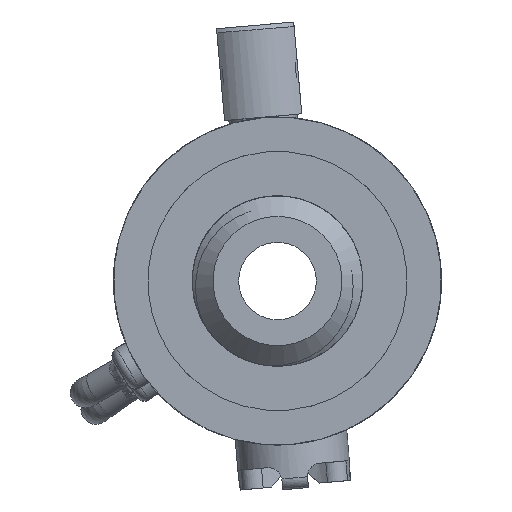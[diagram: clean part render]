
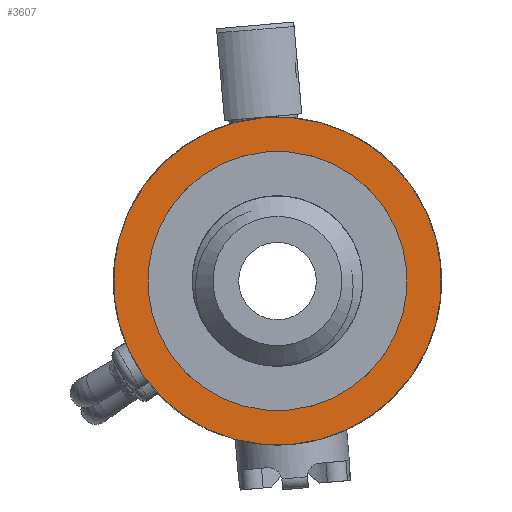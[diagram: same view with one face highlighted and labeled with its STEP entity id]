
A CAD part, left-side view. The second image highlights one B-rep face of the part: STEP entity #3607.
In plain terms, the highlighted planar face has unit normal (-1, 0, 0).
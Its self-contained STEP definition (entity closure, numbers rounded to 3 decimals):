
#204=FACE_BOUND('',#1165,.T.);
#894=FACE_OUTER_BOUND('',#1164,.T.);
#1164=EDGE_LOOP('',(#2832));
#1165=EDGE_LOOP('',(#2833));
#1320=CIRCLE('',#3817,15.05);
#1323=CIRCLE('',#3833,19.05);
#1523=VERTEX_POINT('',#6397);
#1571=VERTEX_POINT('',#7305);
#1927=EDGE_CURVE('',#1523,#1523,#1320,.T.);
#1991=EDGE_CURVE('',#1571,#1571,#1323,.T.);
#2832=ORIENTED_EDGE('',*,*,#1991,.T.);
#2833=ORIENTED_EDGE('',*,*,#1927,.T.);
#3510=PLANE('',#3857);
#3607=ADVANCED_FACE('',(#894,#204),#3510,.T.);
#3817=AXIS2_PLACEMENT_3D('',#6398,#4250,#4251);
#3833=AXIS2_PLACEMENT_3D('',#7306,#4302,#4303);
#3857=AXIS2_PLACEMENT_3D('',#7939,#4367,#4368);
#4250=DIRECTION('center_axis',(1.,0.,0.));
#4251=DIRECTION('ref_axis',(0.,0.996,-0.087));
#4302=DIRECTION('center_axis',(-1.,0.,0.));
#4303=DIRECTION('ref_axis',(0.,0.966,-0.259));
#4367=DIRECTION('center_axis',(-1.,0.,0.));
#4368=DIRECTION('ref_axis',(0.,-0.996,0.087));
#6397=CARTESIAN_POINT('',(-165.,-6.277,99.931));
#6398=CARTESIAN_POINT('Origin',(-165.,8.716,98.619));
#7305=CARTESIAN_POINT('',(-165.,-9.685,103.55));
#7306=CARTESIAN_POINT('Origin',(-165.,8.716,98.619));
#7939=CARTESIAN_POINT('Origin',(-165.,8.724,98.719));
